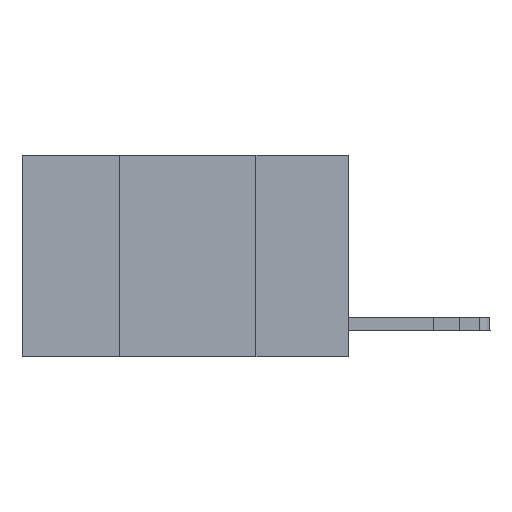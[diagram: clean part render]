
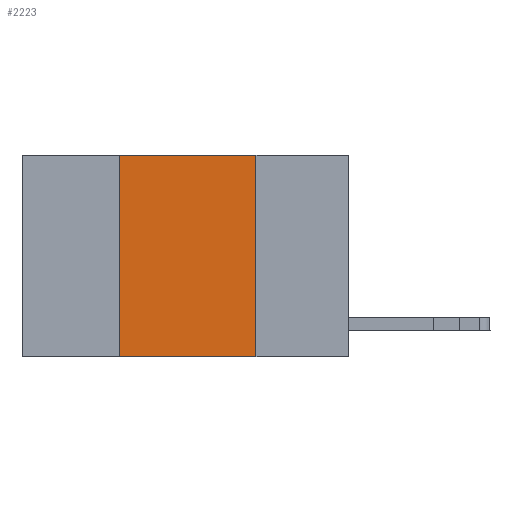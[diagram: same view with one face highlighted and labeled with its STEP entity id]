
A CAD part, left-side view. The second image highlights one B-rep face of the part: STEP entity #2223.
In plain terms, the highlighted planar face has unit normal (-1, 0, 0).
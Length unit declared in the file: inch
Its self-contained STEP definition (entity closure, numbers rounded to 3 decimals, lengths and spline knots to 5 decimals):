
#26 = CARTESIAN_POINT ( 'NONE',  ( 0., 0.17, 0. ) ) ;
#156 = PLANE ( 'NONE',  #20449 ) ;
#2203 = EDGE_CURVE ( 'NONE', #22089, #7442, #11584, .T. ) ;
#2223 = ADVANCED_FACE ( 'NONE', ( #9834 ), #156, .F. ) ;
#2563 = CARTESIAN_POINT ( 'NONE',  ( 0., 0.17, -0.37 ) ) ;
#3228 = EDGE_CURVE ( 'NONE', #10763, #22089, #14271, .T. ) ;
#3802 = CARTESIAN_POINT ( 'NONE',  ( 0., 0.42, -0.37 ) ) ;
#4458 = ORIENTED_EDGE ( 'NONE', *, *, #13102, .F. ) ;
#5267 = LINE ( 'NONE', #20737, #22121 ) ;
#6160 = EDGE_LOOP ( 'NONE', ( #4458, #15074, #11084, #18026 ) ) ;
#7442 = VERTEX_POINT ( 'NONE', #24395 ) ;
#8050 = DIRECTION ( 'NONE',  ( 0., -1., 0. ) ) ;
#8818 = CARTESIAN_POINT ( 'NONE',  ( 0., 0.42, 0. ) ) ;
#9834 = FACE_OUTER_BOUND ( 'NONE', #6160, .T. ) ;
#10763 = VERTEX_POINT ( 'NONE', #3802 ) ;
#11084 = ORIENTED_EDGE ( 'NONE', *, *, #3228, .F. ) ;
#11221 = VECTOR ( 'NONE', #23650, 39.37008 ) ;
#11584 = LINE ( 'NONE', #21405, #14745 ) ;
#12880 = VERTEX_POINT ( 'NONE', #2563 ) ;
#13102 = EDGE_CURVE ( 'NONE', #7442, #12880, #17664, .T. ) ;
#14271 = LINE ( 'NONE', #8818, #20493 ) ;
#14745 = VECTOR ( 'NONE', #8050, 39.37008 ) ;
#15074 = ORIENTED_EDGE ( 'NONE', *, *, #2203, .F. ) ;
#17664 = LINE ( 'NONE', #26, #11221 ) ;
#18026 = ORIENTED_EDGE ( 'NONE', *, *, #22465, .T. ) ;
#18821 = DIRECTION ( 'NONE',  ( 0., -1., 0. ) ) ;
#19713 = DIRECTION ( 'NONE',  ( 1., 0., 0. ) ) ;
#20238 = DIRECTION ( 'NONE',  ( 0., 0., 1. ) ) ;
#20449 = AXIS2_PLACEMENT_3D ( 'NONE', #21284, #19713, #25078 ) ;
#20493 = VECTOR ( 'NONE', #20238, 39.37008 ) ;
#20548 = CARTESIAN_POINT ( 'NONE',  ( 0., 0.42, 0. ) ) ;
#20737 = CARTESIAN_POINT ( 'NONE',  ( 0., 0.6, -0.37 ) ) ;
#21284 = CARTESIAN_POINT ( 'NONE',  ( 0., 0.6, 0. ) ) ;
#21405 = CARTESIAN_POINT ( 'NONE',  ( 0., 0.6, 0. ) ) ;
#22089 = VERTEX_POINT ( 'NONE', #20548 ) ;
#22121 = VECTOR ( 'NONE', #18821, 39.37008 ) ;
#22465 = EDGE_CURVE ( 'NONE', #10763, #12880, #5267, .T. ) ;
#23650 = DIRECTION ( 'NONE',  ( 0., 0., -1. ) ) ;
#24395 = CARTESIAN_POINT ( 'NONE',  ( 0., 0.17, 0. ) ) ;
#25078 = DIRECTION ( 'NONE',  ( 0., 0., -1. ) ) ;
